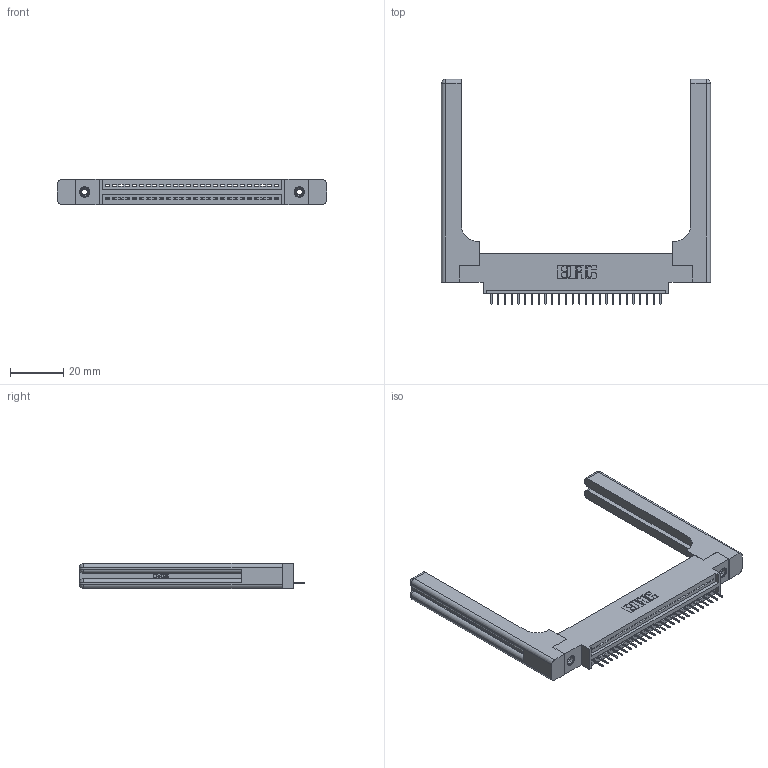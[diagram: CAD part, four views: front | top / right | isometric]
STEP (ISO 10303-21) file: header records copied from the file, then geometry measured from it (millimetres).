
FILE_DESCRIPTION (( 'STEP AP203' ), '1' );
FILE_NAME ('395-026-524-658.STEP', '2019-10-18T09:31:14', ( '' ), ( '' ), 'SwSTEP 2.0', 'SolidWorks 2016', '' );
FILE_SCHEMA (( 'CONFIG_CONTROL_DESIGN' ));
Length unit declared in the file: inch
Products named in the file (5): 345-250-001_345-250-001-102; 345-220-058_345-220-058; 345-292-001_345-293-124; 395-026-524-658; 345 Part_0.170 Offset - 0.156 Dia-TH
Assembly tree (31 placements, depth 2):
  395-026-524-658
    345 Part_0.170 Offset - 0.156 Dia-TH
    345-292-001_345-293-124  x26
    345-250-001_345-250-001-102  x2
    345-220-058_345-220-058  x2
Bounding box: 101.07 x 84.63 x 9.4 mm (x, y, z)
Volume: 17757.2 mm3; surface area: 17181.7 mm2
Topology: 31 solids, 31 shells, 1998 faces, 5699 edges, 3674 vertices
Faces by surface type: plane 1428, cylinder 510, bspline 36, cone 12, sphere 8, torus 4
Entity records: 27110 total; most frequent: CARTESIAN_POINT 5667, ORIENTED_EDGE 4424, DIRECTION 3920, EDGE_CURVE 2212, LINE 1888, VECTOR 1888, VERTEX_POINT 1462, AXIS2_PLACEMENT_3D 1016
